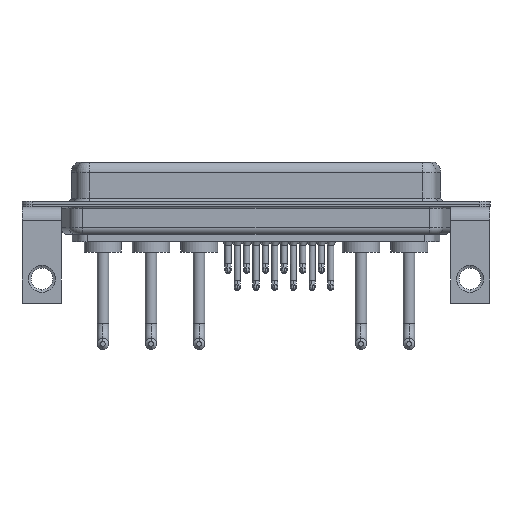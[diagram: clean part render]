
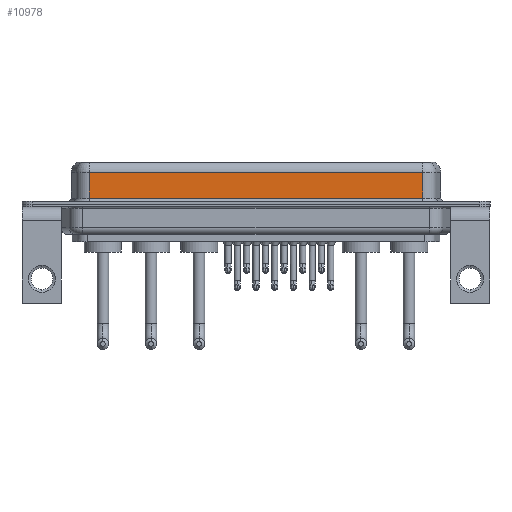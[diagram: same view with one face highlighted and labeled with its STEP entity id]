
A CAD part, front view. The second image highlights one B-rep face of the part: STEP entity #10978.
In plain terms, the highlighted planar face has unit normal (0, -1, 0).
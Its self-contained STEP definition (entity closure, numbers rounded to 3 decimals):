
#329 = CARTESIAN_POINT ( 'NONE',  ( 56.462, -3.95, 4.65 ) ) ;
#338 = LINE ( 'NONE', #6800, #17453 ) ;
#406 = EDGE_CURVE ( 'NONE', #2025, #18037, #16632, .T. ) ;
#545 = AXIS2_PLACEMENT_3D ( 'NONE', #11715, #8530, #18101 ) ;
#1344 = EDGE_CURVE ( 'NONE', #19162, #11517, #11681, .T. ) ;
#2025 = VERTEX_POINT ( 'NONE', #18926 ) ;
#2042 = FACE_OUTER_BOUND ( 'NONE', #14836, .T. ) ;
#3536 = PLANE ( 'NONE',  #545 ) ;
#4018 = CARTESIAN_POINT ( 'NONE',  ( 56.462, -3.95, 6.4 ) ) ;
#5247 = DIRECTION ( 'NONE',  ( 1., 0., 0. ) ) ;
#6800 = CARTESIAN_POINT ( 'NONE',  ( 7.038, -3.95, 6.4 ) ) ;
#6999 = DIRECTION ( 'NONE',  ( -1., 0., 0. ) ) ;
#7234 = ORIENTED_EDGE ( 'NONE', *, *, #20065, .F. ) ;
#7576 = CARTESIAN_POINT ( 'NONE',  ( 56.462, -3.95, 4.65 ) ) ;
#8530 = DIRECTION ( 'NONE',  ( 0., 1., 0. ) ) ;
#9441 = EDGE_CURVE ( 'NONE', #11517, #2025, #338, .T. ) ;
#10570 = CARTESIAN_POINT ( 'NONE',  ( 56.462, -3.95, 0.9 ) ) ;
#10978 = ADVANCED_FACE ( 'NONE', ( #2042 ), #3536, .F. ) ;
#11517 = VERTEX_POINT ( 'NONE', #20541 ) ;
#11681 = LINE ( 'NONE', #329, #13215 ) ;
#11715 = CARTESIAN_POINT ( 'NONE',  ( 56.462, -3.95, 6.4 ) ) ;
#12260 = ORIENTED_EDGE ( 'NONE', *, *, #9441, .T. ) ;
#13215 = VECTOR ( 'NONE', #6999, 1000. ) ;
#13285 = DIRECTION ( 'NONE',  ( 0., 0., -1. ) ) ;
#14336 = VECTOR ( 'NONE', #5247, 1000. ) ;
#14836 = EDGE_LOOP ( 'NONE', ( #7234, #19689, #12260, #20421 ) ) ;
#16632 = LINE ( 'NONE', #10570, #14336 ) ;
#17453 = VECTOR ( 'NONE', #13285, 1000. ) ;
#18037 = VERTEX_POINT ( 'NONE', #18292 ) ;
#18101 = DIRECTION ( 'NONE',  ( 0., 0., 1. ) ) ;
#18292 = CARTESIAN_POINT ( 'NONE',  ( 56.462, -3.95, 0.9 ) ) ;
#18926 = CARTESIAN_POINT ( 'NONE',  ( 7.038, -3.95, 0.9 ) ) ;
#19162 = VERTEX_POINT ( 'NONE', #7576 ) ;
#19689 = ORIENTED_EDGE ( 'NONE', *, *, #1344, .T. ) ;
#19967 = DIRECTION ( 'NONE',  ( 0., 0., -1. ) ) ;
#20065 = EDGE_CURVE ( 'NONE', #19162, #18037, #20070, .T. ) ;
#20070 = LINE ( 'NONE', #4018, #20395 ) ;
#20395 = VECTOR ( 'NONE', #19967, 1000. ) ;
#20421 = ORIENTED_EDGE ( 'NONE', *, *, #406, .T. ) ;
#20541 = CARTESIAN_POINT ( 'NONE',  ( 7.038, -3.95, 4.65 ) ) ;
